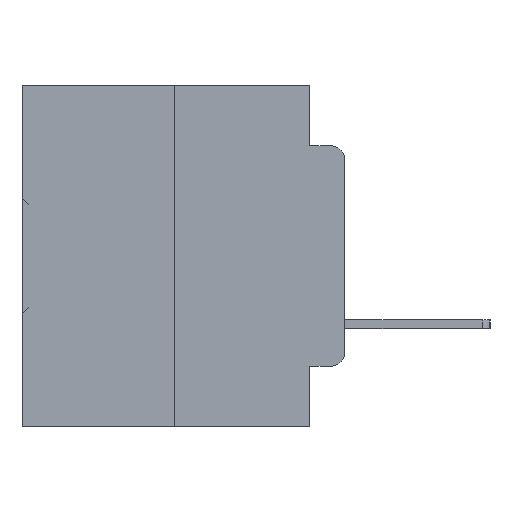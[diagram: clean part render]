
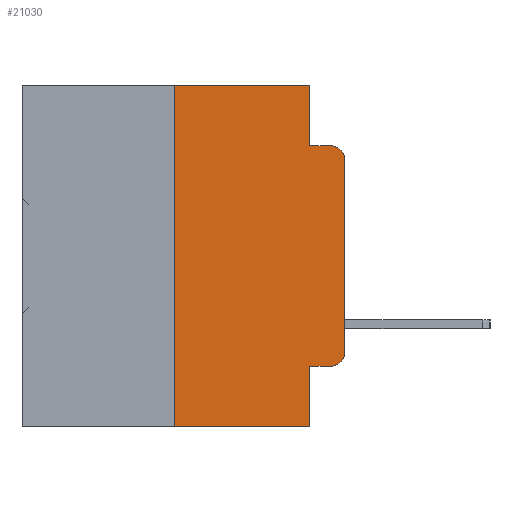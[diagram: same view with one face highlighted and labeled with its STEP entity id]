
A CAD part, left-side view. The second image highlights one B-rep face of the part: STEP entity #21030.
In plain terms, the highlighted planar face has unit normal (-1, 0, 0).
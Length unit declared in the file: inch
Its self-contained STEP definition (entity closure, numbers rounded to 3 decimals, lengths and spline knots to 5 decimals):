
#338 = VERTEX_POINT ( 'NONE', #25721 ) ;
#955 = LINE ( 'NONE', #3299, #7603 ) ;
#1134 = DIRECTION ( 'NONE',  ( 0., 0., -1. ) ) ;
#2058 = DIRECTION ( 'NONE',  ( -1., 0., 0. ) ) ;
#2094 = LINE ( 'NONE', #12363, #16247 ) ;
#2266 = VERTEX_POINT ( 'NONE', #26996 ) ;
#2674 = CARTESIAN_POINT ( 'NONE',  ( 0., 0.473, -0.5 ) ) ;
#2939 = EDGE_CURVE ( 'NONE', #2266, #28548, #20465, .T. ) ;
#3006 = DIRECTION ( 'NONE',  ( 0., -1., 0. ) ) ;
#3215 = CARTESIAN_POINT ( 'NONE',  ( 0., 0.051, -0.4115 ) ) ;
#3299 = CARTESIAN_POINT ( 'NONE',  ( 0., 0.051, -0.4115 ) ) ;
#4317 = PLANE ( 'NONE',  #9338 ) ;
#4378 = CARTESIAN_POINT ( 'NONE',  ( 0., 0., 0. ) ) ;
#4619 = FACE_OUTER_BOUND ( 'NONE', #32519, .T. ) ;
#4831 = EDGE_CURVE ( 'NONE', #338, #28548, #29839, .T. ) ;
#5412 = CARTESIAN_POINT ( 'NONE',  ( 0., 0.02, -0.0885 ) ) ;
#6231 = CARTESIAN_POINT ( 'NONE',  ( 0., 0., -0.3915 ) ) ;
#6248 = DIRECTION ( 'NONE',  ( 0., 0., -1. ) ) ;
#6341 = ORIENTED_EDGE ( 'NONE', *, *, #10964, .T. ) ;
#7048 = CARTESIAN_POINT ( 'NONE',  ( 0., 0.473, 0. ) ) ;
#7183 = DIRECTION ( 'NONE',  ( 0., 0., -1. ) ) ;
#7603 = VECTOR ( 'NONE', #11920, 39.37008 ) ;
#7636 = CARTESIAN_POINT ( 'NONE',  ( 0., 0.02, -0.3915 ) ) ;
#7879 = ORIENTED_EDGE ( 'NONE', *, *, #16929, .T. ) ;
#8220 = VECTOR ( 'NONE', #3006, 39.37008 ) ;
#8274 = ORIENTED_EDGE ( 'NONE', *, *, #8880, .F. ) ;
#8335 = CARTESIAN_POINT ( 'NONE',  ( 0., 0.25, -0.5 ) ) ;
#8609 = EDGE_CURVE ( 'NONE', #31126, #338, #10442, .T. ) ;
#8681 = VECTOR ( 'NONE', #15792, 39.37008 ) ;
#8880 = EDGE_CURVE ( 'NONE', #21294, #12429, #36071, .T. ) ;
#9338 = AXIS2_PLACEMENT_3D ( 'NONE', #7048, #24025, #7183 ) ;
#9550 = ORIENTED_EDGE ( 'NONE', *, *, #29934, .F. ) ;
#9689 = CARTESIAN_POINT ( 'NONE',  ( 0., 0.051, -0.0885 ) ) ;
#10434 = DIRECTION ( 'NONE',  ( 0., 0., -1. ) ) ;
#10442 = LINE ( 'NONE', #4378, #8681 ) ;
#10964 = EDGE_CURVE ( 'NONE', #15245, #33633, #23907, .T. ) ;
#11791 = CARTESIAN_POINT ( 'NONE',  ( 0., 0.051, 0. ) ) ;
#11920 = DIRECTION ( 'NONE',  ( 0., -1., 0. ) ) ;
#12363 = CARTESIAN_POINT ( 'NONE',  ( 0., 0.051, 0. ) ) ;
#12429 = VERTEX_POINT ( 'NONE', #31315 ) ;
#13933 = CIRCLE ( 'NONE', #14687, 0.02 ) ;
#14687 = AXIS2_PLACEMENT_3D ( 'NONE', #7636, #27258, #10434 ) ;
#15044 = EDGE_CURVE ( 'NONE', #26342, #31126, #13933, .T. ) ;
#15245 = VERTEX_POINT ( 'NONE', #8335 ) ;
#15792 = DIRECTION ( 'NONE',  ( 0., 0., 1. ) ) ;
#16247 = VECTOR ( 'NONE', #1134, 39.37008 ) ;
#16260 = CARTESIAN_POINT ( 'NONE',  ( 0., 0.25, 0. ) ) ;
#16929 = EDGE_CURVE ( 'NONE', #34242, #26342, #955, .T. ) ;
#18443 = AXIS2_PLACEMENT_3D ( 'NONE', #18971, #2058, #21781 ) ;
#18797 = EDGE_CURVE ( 'NONE', #34242, #33633, #19808, .T. ) ;
#18971 = CARTESIAN_POINT ( 'NONE',  ( 0., 0.02, -0.1085 ) ) ;
#19808 = LINE ( 'NONE', #11791, #26327 ) ;
#19894 = VECTOR ( 'NONE', #35694, 39.37008 ) ;
#19926 = CARTESIAN_POINT ( 'NONE',  ( 0., 0.473, 0. ) ) ;
#20465 = LINE ( 'NONE', #9689, #33391 ) ;
#21030 = ADVANCED_FACE ( 'NONE', ( #4619 ), #4317, .F. ) ;
#21294 = VERTEX_POINT ( 'NONE', #33364 ) ;
#21351 = ORIENTED_EDGE ( 'NONE', *, *, #8609, .T. ) ;
#21781 = DIRECTION ( 'NONE',  ( 0., 0., -1. ) ) ;
#23098 = CARTESIAN_POINT ( 'NONE',  ( 0., 0.051, -0.5 ) ) ;
#23907 = LINE ( 'NONE', #2674, #30348 ) ;
#24025 = DIRECTION ( 'NONE',  ( 1., 0., 0. ) ) ;
#25181 = DIRECTION ( 'NONE',  ( 0., -1., 0. ) ) ;
#25721 = CARTESIAN_POINT ( 'NONE',  ( 0., 0., -0.1085 ) ) ;
#26327 = VECTOR ( 'NONE', #6248, 39.37008 ) ;
#26342 = VERTEX_POINT ( 'NONE', #35914 ) ;
#26996 = CARTESIAN_POINT ( 'NONE',  ( 0., 0.051, -0.0885 ) ) ;
#27258 = DIRECTION ( 'NONE',  ( -1., 0., 0. ) ) ;
#27294 = LINE ( 'NONE', #16260, #19894 ) ;
#28107 = EDGE_CURVE ( 'NONE', #15245, #21294, #27294, .T. ) ;
#28548 = VERTEX_POINT ( 'NONE', #5412 ) ;
#29251 = ORIENTED_EDGE ( 'NONE', *, *, #18797, .F. ) ;
#29839 = CIRCLE ( 'NONE', #18443, 0.02 ) ;
#29934 = EDGE_CURVE ( 'NONE', #12429, #2266, #2094, .T. ) ;
#30348 = VECTOR ( 'NONE', #25181, 39.37008 ) ;
#30843 = ORIENTED_EDGE ( 'NONE', *, *, #4831, .T. ) ;
#31126 = VERTEX_POINT ( 'NONE', #6231 ) ;
#31315 = CARTESIAN_POINT ( 'NONE',  ( 0., 0.051, 0. ) ) ;
#31552 = ORIENTED_EDGE ( 'NONE', *, *, #15044, .T. ) ;
#32519 = EDGE_LOOP ( 'NONE', ( #21351, #30843, #33055, #9550, #8274, #34962, #6341, #29251, #7879, #31552 ) ) ;
#33055 = ORIENTED_EDGE ( 'NONE', *, *, #2939, .F. ) ;
#33364 = CARTESIAN_POINT ( 'NONE',  ( 0., 0.25, 0. ) ) ;
#33391 = VECTOR ( 'NONE', #34653, 39.37008 ) ;
#33633 = VERTEX_POINT ( 'NONE', #23098 ) ;
#34242 = VERTEX_POINT ( 'NONE', #3215 ) ;
#34653 = DIRECTION ( 'NONE',  ( 0., -1., 0. ) ) ;
#34962 = ORIENTED_EDGE ( 'NONE', *, *, #28107, .F. ) ;
#35694 = DIRECTION ( 'NONE',  ( 0., 0., 1. ) ) ;
#35914 = CARTESIAN_POINT ( 'NONE',  ( 0., 0.02, -0.4115 ) ) ;
#36071 = LINE ( 'NONE', #19926, #8220 ) ;
